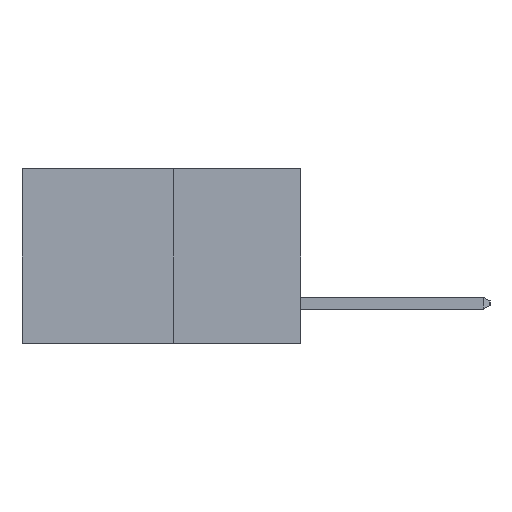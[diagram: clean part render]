
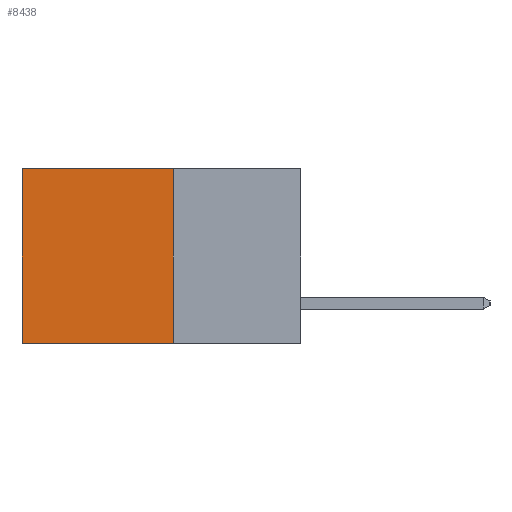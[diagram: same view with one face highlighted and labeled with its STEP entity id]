
A CAD part, left-side view. The second image highlights one B-rep face of the part: STEP entity #8438.
In plain terms, the highlighted planar face has unit normal (-1, 0, 0).
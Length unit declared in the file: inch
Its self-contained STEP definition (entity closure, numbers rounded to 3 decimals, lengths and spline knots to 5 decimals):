
#91 = VECTOR ( 'NONE', #4784, 39.37008 ) ;
#160 = CARTESIAN_POINT ( 'NONE',  ( 0.277, 0.27, -0.37 ) ) ;
#568 = LINE ( 'NONE', #924, #5342 ) ;
#762 = AXIS2_PLACEMENT_3D ( 'NONE', #160, #1219, #7876 ) ;
#924 = CARTESIAN_POINT ( 'NONE',  ( 0.277, 0.27, -0.37 ) ) ;
#1219 = DIRECTION ( 'NONE',  ( 1., 0., 0. ) ) ;
#1772 = CARTESIAN_POINT ( 'NONE',  ( 0.277, 0.27, 0. ) ) ;
#1892 = DIRECTION ( 'NONE',  ( 0., 1., 0. ) ) ;
#2337 = CARTESIAN_POINT ( 'NONE',  ( 0.277, 0.59, -0.37 ) ) ;
#2681 = EDGE_LOOP ( 'NONE', ( #7771, #7792, #7830, #7854 ) ) ;
#2704 = LINE ( 'NONE', #8539, #91 ) ;
#2923 = VERTEX_POINT ( 'NONE', #1772 ) ;
#3099 = CARTESIAN_POINT ( 'NONE',  ( 0.277, 0.59, 0. ) ) ;
#3983 = VERTEX_POINT ( 'NONE', #2337 ) ;
#4026 = PLANE ( 'NONE',  #762 ) ;
#4147 = VECTOR ( 'NONE', #5206, 39.37008 ) ;
#4784 = DIRECTION ( 'NONE',  ( 0., 0., -1. ) ) ;
#5206 = DIRECTION ( 'NONE',  ( 0., 1., 0. ) ) ;
#5342 = VECTOR ( 'NONE', #1892, 39.37008 ) ;
#5378 = VERTEX_POINT ( 'NONE', #9851 ) ;
#6045 = VECTOR ( 'NONE', #9304, 39.37008 ) ;
#6176 = CARTESIAN_POINT ( 'NONE',  ( 0.277, 0.27, 0. ) ) ;
#6619 = CARTESIAN_POINT ( 'NONE',  ( 0.277, 0.59, -0.37 ) ) ;
#7020 = LINE ( 'NONE', #6176, #4147 ) ;
#7771 = ORIENTED_EDGE ( 'NONE', *, *, #11311, .T. ) ;
#7792 = ORIENTED_EDGE ( 'NONE', *, *, #8905, .F. ) ;
#7830 = ORIENTED_EDGE ( 'NONE', *, *, #8297, .F. ) ;
#7854 = ORIENTED_EDGE ( 'NONE', *, *, #8607, .T. ) ;
#7876 = DIRECTION ( 'NONE',  ( 0., 0., -1. ) ) ;
#8297 = EDGE_CURVE ( 'NONE', #2923, #5378, #2704, .T. ) ;
#8438 = ADVANCED_FACE ( 'NONE', ( #8448 ), #4026, .F. ) ;
#8448 = FACE_OUTER_BOUND ( 'NONE', #2681, .T. ) ;
#8523 = LINE ( 'NONE', #6619, #6045 ) ;
#8539 = CARTESIAN_POINT ( 'NONE',  ( 0.277, 0.27, -0.37 ) ) ;
#8607 = EDGE_CURVE ( 'NONE', #2923, #10302, #7020, .T. ) ;
#8905 = EDGE_CURVE ( 'NONE', #5378, #3983, #568, .T. ) ;
#9304 = DIRECTION ( 'NONE',  ( 0., 0., -1. ) ) ;
#9851 = CARTESIAN_POINT ( 'NONE',  ( 0.277, 0.27, -0.37 ) ) ;
#10302 = VERTEX_POINT ( 'NONE', #3099 ) ;
#11311 = EDGE_CURVE ( 'NONE', #10302, #3983, #8523, .T. ) ;
